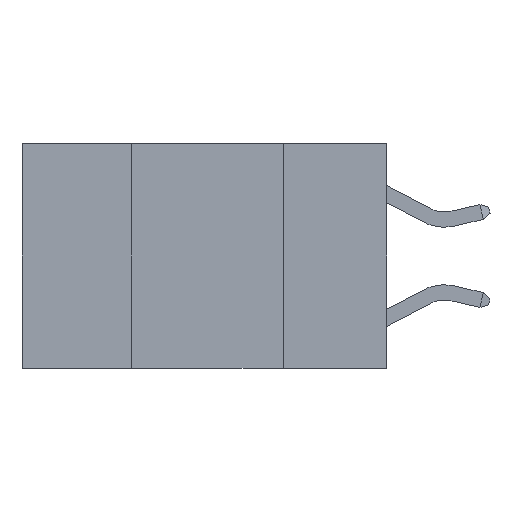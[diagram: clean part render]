
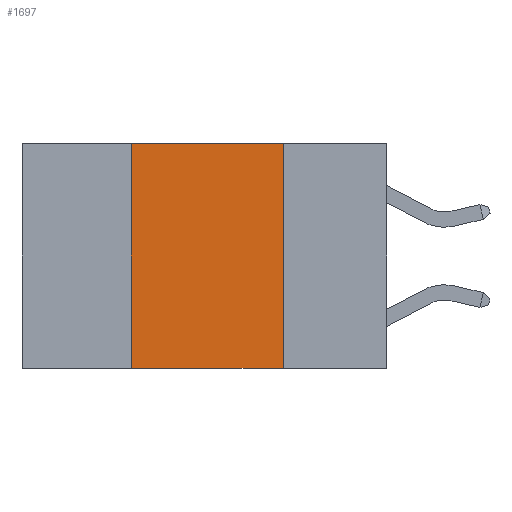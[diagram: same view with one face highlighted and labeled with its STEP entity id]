
A CAD part, left-side view. The second image highlights one B-rep face of the part: STEP entity #1697.
In plain terms, the highlighted planar face has unit normal (-1, 0, 0).
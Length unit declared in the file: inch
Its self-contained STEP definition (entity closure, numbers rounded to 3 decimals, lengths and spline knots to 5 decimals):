
#206 = LINE ( 'NONE', #1761, #4746 ) ;
#218 = VECTOR ( 'NONE', #2972, 39.37008 ) ;
#268 = CARTESIAN_POINT ( 'NONE',  ( 0., 0.42, 0. ) ) ;
#773 = PLANE ( 'NONE',  #3870 ) ;
#807 = VERTEX_POINT ( 'NONE', #4668 ) ;
#868 = DIRECTION ( 'NONE',  ( 1., 0., 0. ) ) ;
#1396 = EDGE_CURVE ( 'NONE', #3401, #807, #4468, .T. ) ;
#1697 = ADVANCED_FACE ( 'NONE', ( #7778 ), #773, .F. ) ;
#1761 = CARTESIAN_POINT ( 'NONE',  ( 0., 0.6, -0.37 ) ) ;
#2148 = ORIENTED_EDGE ( 'NONE', *, *, #2727, .F. ) ;
#2214 = DIRECTION ( 'NONE',  ( 0., 0., -1. ) ) ;
#2305 = CARTESIAN_POINT ( 'NONE',  ( 0., 0.17, 0. ) ) ;
#2398 = VERTEX_POINT ( 'NONE', #7911 ) ;
#2727 = EDGE_CURVE ( 'NONE', #807, #2398, #6490, .T. ) ;
#2739 = CARTESIAN_POINT ( 'NONE',  ( 0., 0.42, 0. ) ) ;
#2972 = DIRECTION ( 'NONE',  ( 0., 0., 1. ) ) ;
#3372 = EDGE_LOOP ( 'NONE', ( #2148, #7317, #7658, #7436 ) ) ;
#3401 = VERTEX_POINT ( 'NONE', #2739 ) ;
#3756 = LINE ( 'NONE', #268, #218 ) ;
#3870 = AXIS2_PLACEMENT_3D ( 'NONE', #4262, #868, #7058 ) ;
#4024 = EDGE_CURVE ( 'NONE', #4609, #2398, #206, .T. ) ;
#4262 = CARTESIAN_POINT ( 'NONE',  ( 0., 0.6, 0. ) ) ;
#4468 = LINE ( 'NONE', #5795, #8461 ) ;
#4609 = VERTEX_POINT ( 'NONE', #8069 ) ;
#4668 = CARTESIAN_POINT ( 'NONE',  ( 0., 0.17, 0. ) ) ;
#4746 = VECTOR ( 'NONE', #7264, 39.37008 ) ;
#4861 = EDGE_CURVE ( 'NONE', #4609, #3401, #3756, .T. ) ;
#5795 = CARTESIAN_POINT ( 'NONE',  ( 0., 0.6, 0. ) ) ;
#6490 = LINE ( 'NONE', #2305, #7616 ) ;
#7058 = DIRECTION ( 'NONE',  ( 0., 0., -1. ) ) ;
#7128 = DIRECTION ( 'NONE',  ( 0., -1., 0. ) ) ;
#7264 = DIRECTION ( 'NONE',  ( 0., -1., 0. ) ) ;
#7317 = ORIENTED_EDGE ( 'NONE', *, *, #1396, .F. ) ;
#7436 = ORIENTED_EDGE ( 'NONE', *, *, #4024, .T. ) ;
#7616 = VECTOR ( 'NONE', #2214, 39.37008 ) ;
#7658 = ORIENTED_EDGE ( 'NONE', *, *, #4861, .F. ) ;
#7778 = FACE_OUTER_BOUND ( 'NONE', #3372, .T. ) ;
#7911 = CARTESIAN_POINT ( 'NONE',  ( 0., 0.17, -0.37 ) ) ;
#8069 = CARTESIAN_POINT ( 'NONE',  ( 0., 0.42, -0.37 ) ) ;
#8461 = VECTOR ( 'NONE', #7128, 39.37008 ) ;
